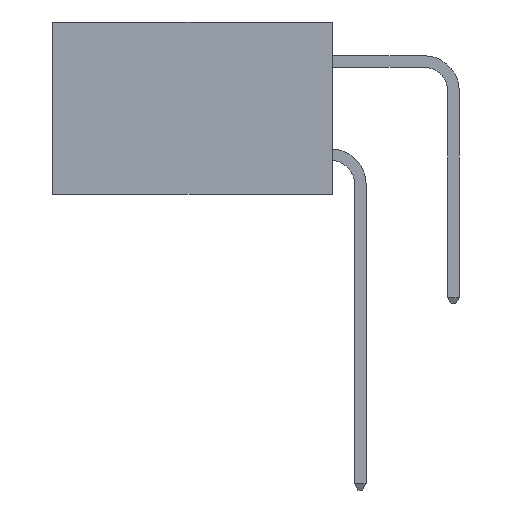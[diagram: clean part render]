
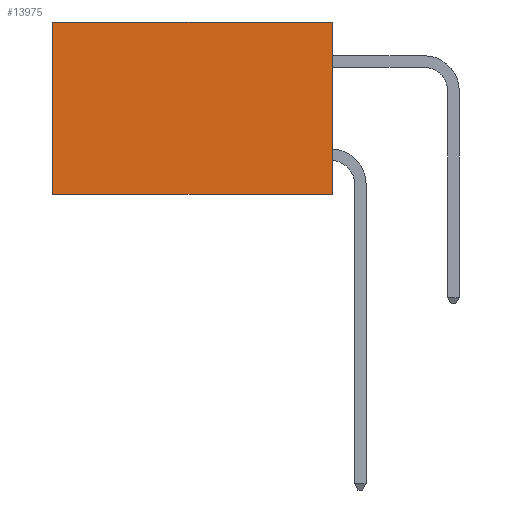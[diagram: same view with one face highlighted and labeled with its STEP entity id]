
A CAD part, left-side view. The second image highlights one B-rep face of the part: STEP entity #13975.
In plain terms, the highlighted planar face has unit normal (-1, 0, 0).
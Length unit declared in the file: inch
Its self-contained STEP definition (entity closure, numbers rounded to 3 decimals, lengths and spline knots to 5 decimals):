
#395 = CARTESIAN_POINT ( 'NONE',  ( 0.2615, 0.6, -0.37 ) ) ;
#1443 = VERTEX_POINT ( 'NONE', #10561 ) ;
#2352 = ORIENTED_EDGE ( 'NONE', *, *, #11422, .F. ) ;
#2389 = VECTOR ( 'NONE', #16442, 39.37008 ) ;
#2954 = LINE ( 'NONE', #16626, #2389 ) ;
#3281 = VERTEX_POINT ( 'NONE', #19484 ) ;
#3289 = CARTESIAN_POINT ( 'NONE',  ( 0.2615, 0., -0.37 ) ) ;
#3596 = CARTESIAN_POINT ( 'NONE',  ( 0.2615, 0., 0. ) ) ;
#3712 = DIRECTION ( 'NONE',  ( 0., 1., 0. ) ) ;
#3954 = FACE_OUTER_BOUND ( 'NONE', #4937, .T. ) ;
#4917 = VECTOR ( 'NONE', #3712, 39.37008 ) ;
#4937 = EDGE_LOOP ( 'NONE', ( #18489, #2352, #10334, #21636 ) ) ;
#4985 = LINE ( 'NONE', #3596, #17823 ) ;
#5087 = VERTEX_POINT ( 'NONE', #6683 ) ;
#5122 = PLANE ( 'NONE',  #17974 ) ;
#6683 = CARTESIAN_POINT ( 'NONE',  ( 0.2615, 0.6, -0.37 ) ) ;
#7204 = EDGE_CURVE ( 'NONE', #3281, #7459, #2954, .T. ) ;
#7459 = VERTEX_POINT ( 'NONE', #13977 ) ;
#10183 = EDGE_CURVE ( 'NONE', #3281, #1443, #4985, .T. ) ;
#10334 = ORIENTED_EDGE ( 'NONE', *, *, #7204, .F. ) ;
#10561 = CARTESIAN_POINT ( 'NONE',  ( 0.2615, 0.6, 0. ) ) ;
#11422 = EDGE_CURVE ( 'NONE', #7459, #5087, #14764, .T. ) ;
#12253 = EDGE_CURVE ( 'NONE', #1443, #5087, #20821, .T. ) ;
#13779 = DIRECTION ( 'NONE',  ( 1., 0., 0. ) ) ;
#13975 = ADVANCED_FACE ( 'NONE', ( #3954 ), #5122, .F. ) ;
#13977 = CARTESIAN_POINT ( 'NONE',  ( 0.2615, 0., -0.37 ) ) ;
#14153 = DIRECTION ( 'NONE',  ( 0., 1., 0. ) ) ;
#14456 = DIRECTION ( 'NONE',  ( 0., 0., -1. ) ) ;
#14764 = LINE ( 'NONE', #17741, #4917 ) ;
#15575 = VECTOR ( 'NONE', #14456, 39.37008 ) ;
#16442 = DIRECTION ( 'NONE',  ( 0., 0., -1. ) ) ;
#16626 = CARTESIAN_POINT ( 'NONE',  ( 0.2615, 0., -0.37 ) ) ;
#17327 = DIRECTION ( 'NONE',  ( 0., 0., -1. ) ) ;
#17741 = CARTESIAN_POINT ( 'NONE',  ( 0.2615, 0., -0.37 ) ) ;
#17823 = VECTOR ( 'NONE', #14153, 39.37008 ) ;
#17974 = AXIS2_PLACEMENT_3D ( 'NONE', #3289, #13779, #17327 ) ;
#18489 = ORIENTED_EDGE ( 'NONE', *, *, #12253, .T. ) ;
#19484 = CARTESIAN_POINT ( 'NONE',  ( 0.2615, 0., 0. ) ) ;
#20821 = LINE ( 'NONE', #395, #15575 ) ;
#21636 = ORIENTED_EDGE ( 'NONE', *, *, #10183, .T. ) ;
